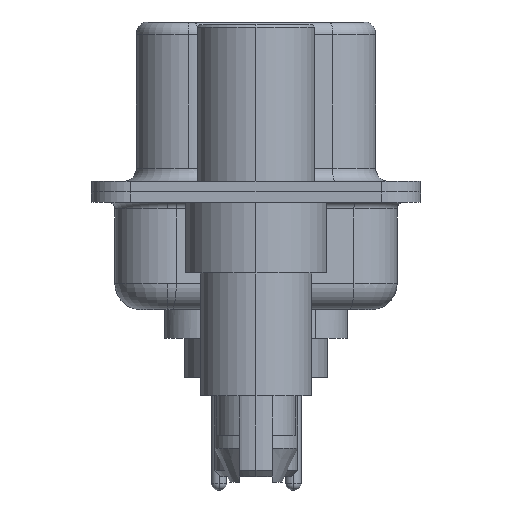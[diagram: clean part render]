
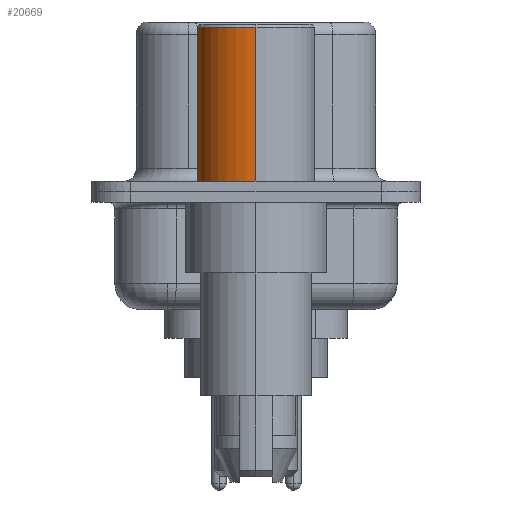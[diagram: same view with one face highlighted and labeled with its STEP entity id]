
A CAD part, left-side view. The second image highlights one B-rep face of the part: STEP entity #20669.
In plain terms, the highlighted cylindrical face has radius 2.25 mm (diameter 4.5 mm), a partial arc.
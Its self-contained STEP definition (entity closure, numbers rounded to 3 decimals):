
#308 = ORIENTED_EDGE ( 'NONE', *, *, #15029, .F. ) ;
#489 = CARTESIAN_POINT ( 'NONE',  ( 2.25, 0., 0.4 ) ) ;
#1252 = CIRCLE ( 'NONE', #14471, 2.25 ) ;
#1722 = DIRECTION ( 'NONE',  ( 0., 0., 1. ) ) ;
#1782 = CIRCLE ( 'NONE', #8995, 2.25 ) ;
#2299 = VECTOR ( 'NONE', #8568, 1000. ) ;
#6113 = VERTEX_POINT ( 'NONE', #18867 ) ;
#6707 = LINE ( 'NONE', #6986, #14912 ) ;
#6967 = CARTESIAN_POINT ( 'NONE',  ( 0., 0., 0.4 ) ) ;
#6986 = CARTESIAN_POINT ( 'NONE',  ( 2.25, 0., 0.581 ) ) ;
#7104 = FACE_OUTER_BOUND ( 'NONE', #11675, .T. ) ;
#7120 = CARTESIAN_POINT ( 'NONE',  ( 0., 0., 6.3 ) ) ;
#7175 = DIRECTION ( 'NONE',  ( 1., 0., 0. ) ) ;
#8568 = DIRECTION ( 'NONE',  ( 0., 0., 1. ) ) ;
#8643 = DIRECTION ( 'NONE',  ( 1., 0., 0. ) ) ;
#8774 = DIRECTION ( 'NONE',  ( 1., 0., 0. ) ) ;
#8995 = AXIS2_PLACEMENT_3D ( 'NONE', #6967, #18253, #8643 ) ;
#9785 = ORIENTED_EDGE ( 'NONE', *, *, #14991, .T. ) ;
#10428 = CYLINDRICAL_SURFACE ( 'NONE', #17625, 2.25 ) ;
#11675 = EDGE_LOOP ( 'NONE', ( #12548, #9785, #308, #17935 ) ) ;
#12548 = ORIENTED_EDGE ( 'NONE', *, *, #14995, .T. ) ;
#12877 = CARTESIAN_POINT ( 'NONE',  ( 2.25, 0., 6.3 ) ) ;
#13294 = VERTEX_POINT ( 'NONE', #16420 ) ;
#14471 = AXIS2_PLACEMENT_3D ( 'NONE', #7120, #18384, #8774 ) ;
#14776 = VERTEX_POINT ( 'NONE', #12877 ) ;
#14806 = EDGE_CURVE ( 'NONE', #18464, #14776, #6707, .T. ) ;
#14912 = VECTOR ( 'NONE', #1722, 1000. ) ;
#14991 = EDGE_CURVE ( 'NONE', #6113, #13294, #15168, .T. ) ;
#14995 = EDGE_CURVE ( 'NONE', #18464, #6113, #1782, .T. ) ;
#15029 = EDGE_CURVE ( 'NONE', #14776, #13294, #1252, .T. ) ;
#15168 = LINE ( 'NONE', #19716, #2299 ) ;
#15412 = DIRECTION ( 'NONE',  ( 0., 0., 1. ) ) ;
#16420 = CARTESIAN_POINT ( 'NONE',  ( -2.25, 0., 6.3 ) ) ;
#16993 = CARTESIAN_POINT ( 'NONE',  ( 0., 0., 0.581 ) ) ;
#17625 = AXIS2_PLACEMENT_3D ( 'NONE', #16993, #15412, #7175 ) ;
#17935 = ORIENTED_EDGE ( 'NONE', *, *, #14806, .F. ) ;
#18253 = DIRECTION ( 'NONE',  ( 0., 0., 1. ) ) ;
#18384 = DIRECTION ( 'NONE',  ( 0., 0., 1. ) ) ;
#18464 = VERTEX_POINT ( 'NONE', #489 ) ;
#18867 = CARTESIAN_POINT ( 'NONE',  ( -2.25, 0., 0.4 ) ) ;
#19716 = CARTESIAN_POINT ( 'NONE',  ( -2.25, 0., 0.581 ) ) ;
#20669 = ADVANCED_FACE ( 'NONE', ( #7104 ), #10428, .T. ) ;
